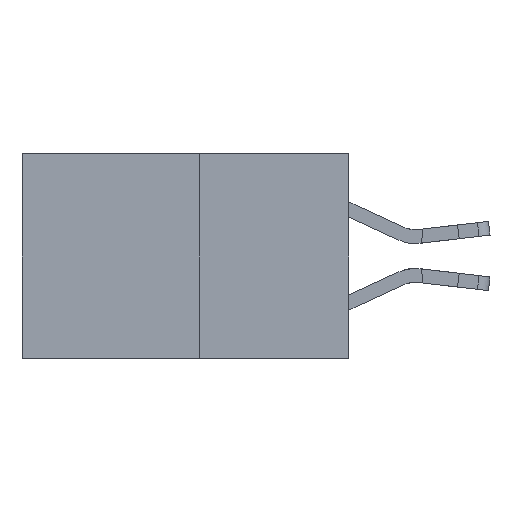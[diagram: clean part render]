
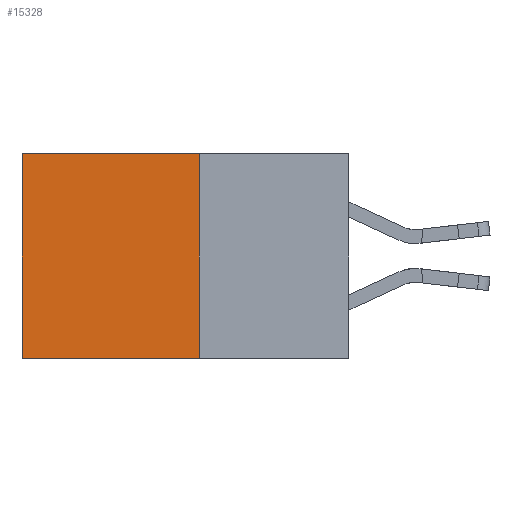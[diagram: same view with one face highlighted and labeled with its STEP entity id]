
A CAD part, left-side view. The second image highlights one B-rep face of the part: STEP entity #15328.
In plain terms, the highlighted planar face has unit normal (-1, 0, 0).
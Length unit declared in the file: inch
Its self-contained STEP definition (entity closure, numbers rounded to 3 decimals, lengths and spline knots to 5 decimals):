
#699 = DIRECTION ( 'NONE',  ( 0., 0., -1. ) ) ;
#753 = CARTESIAN_POINT ( 'NONE',  ( 0.277, 0.59, 0. ) ) ;
#1098 = ORIENTED_EDGE ( 'NONE', *, *, #23261, .F. ) ;
#1380 = CARTESIAN_POINT ( 'NONE',  ( 0.277, 0.59, -0.37 ) ) ;
#2026 = VERTEX_POINT ( 'NONE', #19627 ) ;
#2349 = VECTOR ( 'NONE', #3390, 39.37008 ) ;
#3390 = DIRECTION ( 'NONE',  ( 0., 1., 0. ) ) ;
#4476 = LINE ( 'NONE', #25477, #20451 ) ;
#5531 = PLANE ( 'NONE',  #9542 ) ;
#6372 = CARTESIAN_POINT ( 'NONE',  ( 0.277, 0.27, 0. ) ) ;
#6783 = VECTOR ( 'NONE', #8484, 39.37008 ) ;
#7342 = ORIENTED_EDGE ( 'NONE', *, *, #20632, .T. ) ;
#7659 = DIRECTION ( 'NONE',  ( 1., 0., 0. ) ) ;
#7759 = EDGE_CURVE ( 'NONE', #19631, #2026, #4476, .T. ) ;
#8484 = DIRECTION ( 'NONE',  ( 0., 1., 0. ) ) ;
#8943 = ORIENTED_EDGE ( 'NONE', *, *, #23287, .T. ) ;
#9375 = FACE_OUTER_BOUND ( 'NONE', #24663, .T. ) ;
#9542 = AXIS2_PLACEMENT_3D ( 'NONE', #26091, #7659, #22140 ) ;
#11654 = LINE ( 'NONE', #6372, #6783 ) ;
#12799 = LINE ( 'NONE', #1380, #18391 ) ;
#13814 = CARTESIAN_POINT ( 'NONE',  ( 0.277, 0.27, -0.37 ) ) ;
#13905 = DIRECTION ( 'NONE',  ( 0., 0., -1. ) ) ;
#15328 = ADVANCED_FACE ( 'NONE', ( #9375 ), #5531, .F. ) ;
#17789 = ORIENTED_EDGE ( 'NONE', *, *, #7759, .F. ) ;
#18351 = CARTESIAN_POINT ( 'NONE',  ( 0.277, 0.27, 0. ) ) ;
#18391 = VECTOR ( 'NONE', #13905, 39.37008 ) ;
#19034 = LINE ( 'NONE', #13814, #2349 ) ;
#19627 = CARTESIAN_POINT ( 'NONE',  ( 0.277, 0.27, -0.37 ) ) ;
#19631 = VERTEX_POINT ( 'NONE', #18351 ) ;
#20222 = VERTEX_POINT ( 'NONE', #23756 ) ;
#20451 = VECTOR ( 'NONE', #699, 39.37008 ) ;
#20632 = EDGE_CURVE ( 'NONE', #19631, #21459, #11654, .T. ) ;
#21459 = VERTEX_POINT ( 'NONE', #753 ) ;
#22140 = DIRECTION ( 'NONE',  ( 0., 0., -1. ) ) ;
#23261 = EDGE_CURVE ( 'NONE', #2026, #20222, #19034, .T. ) ;
#23287 = EDGE_CURVE ( 'NONE', #21459, #20222, #12799, .T. ) ;
#23756 = CARTESIAN_POINT ( 'NONE',  ( 0.277, 0.59, -0.37 ) ) ;
#24663 = EDGE_LOOP ( 'NONE', ( #8943, #1098, #17789, #7342 ) ) ;
#25477 = CARTESIAN_POINT ( 'NONE',  ( 0.277, 0.27, -0.37 ) ) ;
#26091 = CARTESIAN_POINT ( 'NONE',  ( 0.277, 0.27, -0.37 ) ) ;
